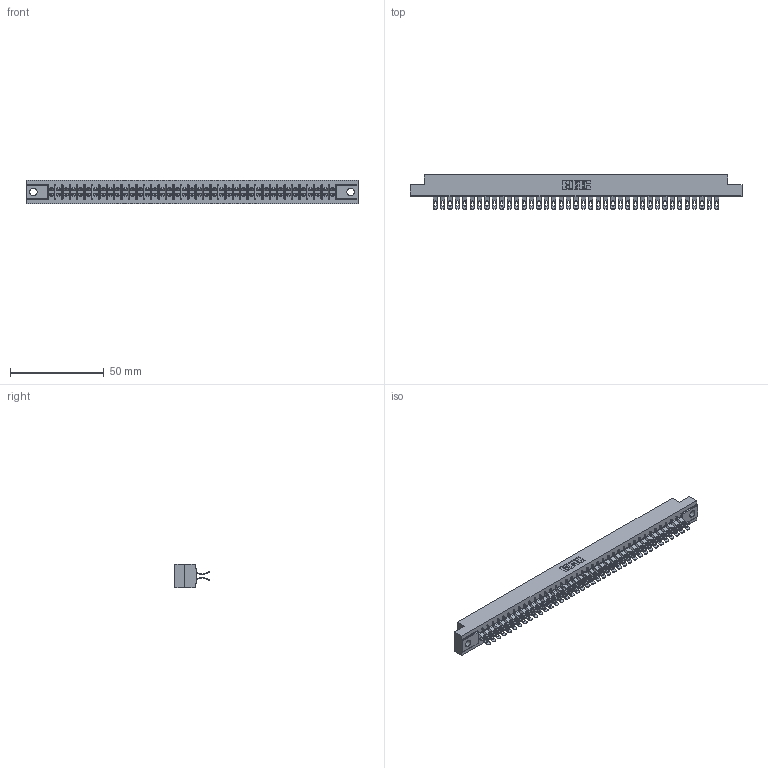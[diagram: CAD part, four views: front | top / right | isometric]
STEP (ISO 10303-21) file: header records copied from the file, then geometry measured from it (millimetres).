
FILE_DESCRIPTION (( 'STEP AP203' ), '1' );
FILE_NAME ('355-078-555-204.STEP', '2019-09-13T14:01:55', ( '' ), ( '' ), 'SwSTEP 2.0', 'SolidWorks 2016', '' );
FILE_SCHEMA (( 'CONFIG_CONTROL_DESIGN' ));
Length unit declared in the file: inch
Products named in the file (3): 355-078-555-204; 305 Part_.156 Dia; 305-290-001_555
Assembly tree (79 placements, depth 2):
  355-078-555-204
    305 Part_.156 Dia
    305-290-001_555  x78
Bounding box: 177.55 x 18.41 x 12.7 mm (x, y, z)
Volume: 18622.6 mm3; surface area: 24943.2 mm2
Topology: 79 solids, 79 shells, 5278 faces, 15757 edges, 10294 vertices
Faces by surface type: plane 2578, cylinder 2544, sphere 156
Entity records: 43634 total; most frequent: CARTESIAN_POINT 7243, ORIENTED_EDGE 7178, DIRECTION 6995, EDGE_CURVE 3589, VECTOR 2887, LINE 2887, VERTEX_POINT 2286, AXIS2_PLACEMENT_3D 2054
